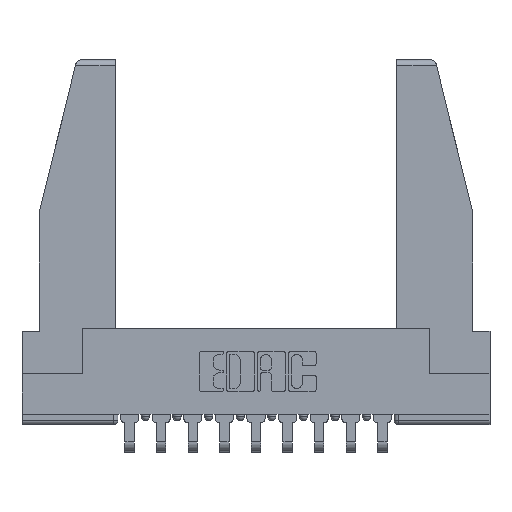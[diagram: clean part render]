
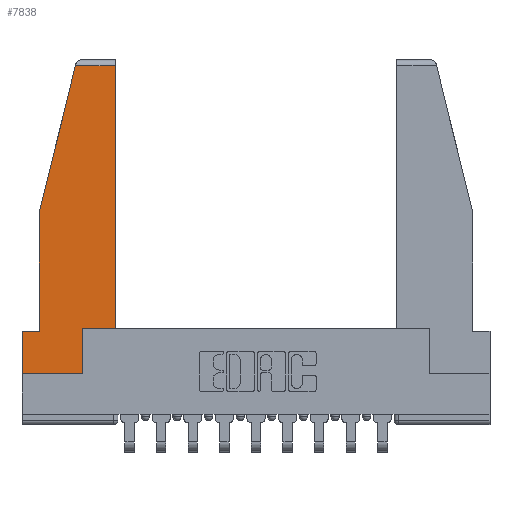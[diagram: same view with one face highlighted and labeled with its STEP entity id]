
A CAD part, top view. The second image highlights one B-rep face of the part: STEP entity #7838.
In plain terms, the highlighted planar face has unit normal (0, 0, 1).
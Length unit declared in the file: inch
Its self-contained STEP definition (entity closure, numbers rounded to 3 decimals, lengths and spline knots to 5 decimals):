
#141 = ORIENTED_EDGE ( 'NONE', *, *, #9137, .T. ) ;
#156 = EDGE_CURVE ( 'NONE', #13078, #12879, #3080, .T. ) ;
#285 = VECTOR ( 'NONE', #3244, 39.37008 ) ;
#340 = CARTESIAN_POINT ( 'NONE',  ( 0.461, 0.223, 0. ) ) ;
#392 = DIRECTION ( 'NONE',  ( 0., 1., 0. ) ) ;
#394 = LINE ( 'NONE', #11386, #6081 ) ;
#431 = CARTESIAN_POINT ( 'NONE',  ( 0.086, 0.8, 0. ) ) ;
#716 = VECTOR ( 'NONE', #1109, 39.37008 ) ;
#779 = CARTESIAN_POINT ( 'NONE',  ( 0., 0.21, 0. ) ) ;
#1109 = DIRECTION ( 'NONE',  ( 0., 1., 0. ) ) ;
#1181 = ORIENTED_EDGE ( 'NONE', *, *, #1972, .T. ) ;
#1295 = LINE ( 'NONE', #3184, #9946 ) ;
#1861 = AXIS2_PLACEMENT_3D ( 'NONE', #2336, #12342, #5687 ) ;
#1972 = EDGE_CURVE ( 'NONE', #10915, #4563, #11006, .T. ) ;
#2336 = CARTESIAN_POINT ( 'NONE',  ( 0., 0., 0. ) ) ;
#2688 = CARTESIAN_POINT ( 'NONE',  ( 0.086, 0.21, 0. ) ) ;
#2776 = CARTESIAN_POINT ( 'NONE',  ( 0.461, 0.223, 0. ) ) ;
#2972 = VERTEX_POINT ( 'NONE', #431 ) ;
#3047 = LINE ( 'NONE', #11991, #3213 ) ;
#3080 = LINE ( 'NONE', #779, #3450 ) ;
#3136 = VERTEX_POINT ( 'NONE', #8514 ) ;
#3184 = CARTESIAN_POINT ( 'NONE',  ( 0., 1.52, 0. ) ) ;
#3213 = VECTOR ( 'NONE', #5344, 39.37008 ) ;
#3244 = DIRECTION ( 'NONE',  ( 0., -1., 0. ) ) ;
#3310 = EDGE_LOOP ( 'NONE', ( #1181, #7034, #141, #14046, #4248, #3653, #4842, #4186, #4631 ) ) ;
#3450 = VECTOR ( 'NONE', #9692, 39.37008 ) ;
#3493 = DIRECTION ( 'NONE',  ( -0.239, -0.971, 0. ) ) ;
#3597 = CARTESIAN_POINT ( 'NONE',  ( 0.297, 0., 0. ) ) ;
#3653 = ORIENTED_EDGE ( 'NONE', *, *, #12987, .T. ) ;
#4054 = DIRECTION ( 'NONE',  ( -1., 0., 0. ) ) ;
#4186 = ORIENTED_EDGE ( 'NONE', *, *, #14027, .T. ) ;
#4248 = ORIENTED_EDGE ( 'NONE', *, *, #156, .T. ) ;
#4563 = VERTEX_POINT ( 'NONE', #13587 ) ;
#4631 = ORIENTED_EDGE ( 'NONE', *, *, #7693, .T. ) ;
#4842 = ORIENTED_EDGE ( 'NONE', *, *, #12642, .T. ) ;
#5292 = FACE_OUTER_BOUND ( 'NONE', #3310, .T. ) ;
#5344 = DIRECTION ( 'NONE',  ( 1., 0., 0. ) ) ;
#5426 = CARTESIAN_POINT ( 'NONE',  ( 0.086, 0.8, 0. ) ) ;
#5687 = DIRECTION ( 'NONE',  ( 1., 0., 0. ) ) ;
#5739 = LINE ( 'NONE', #14286, #12345 ) ;
#5791 = CARTESIAN_POINT ( 'NONE',  ( 0., 0.21, 0. ) ) ;
#5845 = DIRECTION ( 'NONE',  ( 0., -1., 0. ) ) ;
#6081 = VECTOR ( 'NONE', #5845, 39.37008 ) ;
#6319 = VECTOR ( 'NONE', #392, 39.37008 ) ;
#6758 = PLANE ( 'NONE',  #1861 ) ;
#6982 = CARTESIAN_POINT ( 'NONE',  ( 0.271, 1.55, 0. ) ) ;
#7034 = ORIENTED_EDGE ( 'NONE', *, *, #8871, .T. ) ;
#7693 = EDGE_CURVE ( 'NONE', #11887, #10915, #3047, .T. ) ;
#7838 = ADVANCED_FACE ( 'NONE', ( #5292 ), #6758, .T. ) ;
#7918 = VERTEX_POINT ( 'NONE', #12638 ) ;
#8059 = VECTOR ( 'NONE', #3493, 39.37008 ) ;
#8302 = EDGE_CURVE ( 'NONE', #2972, #13078, #12934, .T. ) ;
#8514 = CARTESIAN_POINT ( 'NONE',  ( 0.2636, 1.52, 0. ) ) ;
#8871 = EDGE_CURVE ( 'NONE', #4563, #3136, #1295, .T. ) ;
#8917 = LINE ( 'NONE', #6982, #8059 ) ;
#9137 = EDGE_CURVE ( 'NONE', #3136, #2972, #8917, .T. ) ;
#9377 = LINE ( 'NONE', #9834, #716 ) ;
#9628 = DIRECTION ( 'NONE',  ( 1., 0., 0. ) ) ;
#9692 = DIRECTION ( 'NONE',  ( -1., 0., 0. ) ) ;
#9834 = CARTESIAN_POINT ( 'NONE',  ( 0.297, 0., 0. ) ) ;
#9946 = VECTOR ( 'NONE', #4054, 39.37008 ) ;
#10915 = VERTEX_POINT ( 'NONE', #2776 ) ;
#11006 = LINE ( 'NONE', #340, #6319 ) ;
#11296 = VERTEX_POINT ( 'NONE', #3597 ) ;
#11386 = CARTESIAN_POINT ( 'NONE',  ( 0., 0.21, 0. ) ) ;
#11887 = VERTEX_POINT ( 'NONE', #12303 ) ;
#11991 = CARTESIAN_POINT ( 'NONE',  ( 0.297, 0.223, 0. ) ) ;
#12303 = CARTESIAN_POINT ( 'NONE',  ( 0.297, 0.223, 0. ) ) ;
#12342 = DIRECTION ( 'NONE',  ( 0., 0., 1. ) ) ;
#12345 = VECTOR ( 'NONE', #9628, 39.37008 ) ;
#12638 = CARTESIAN_POINT ( 'NONE',  ( 0., 0., 0. ) ) ;
#12642 = EDGE_CURVE ( 'NONE', #7918, #11296, #5739, .T. ) ;
#12879 = VERTEX_POINT ( 'NONE', #5791 ) ;
#12934 = LINE ( 'NONE', #5426, #285 ) ;
#12987 = EDGE_CURVE ( 'NONE', #12879, #7918, #394, .T. ) ;
#13078 = VERTEX_POINT ( 'NONE', #2688 ) ;
#13587 = CARTESIAN_POINT ( 'NONE',  ( 0.461, 1.52, 0. ) ) ;
#14027 = EDGE_CURVE ( 'NONE', #11296, #11887, #9377, .T. ) ;
#14046 = ORIENTED_EDGE ( 'NONE', *, *, #8302, .T. ) ;
#14286 = CARTESIAN_POINT ( 'NONE',  ( 0., 0., 0. ) ) ;
